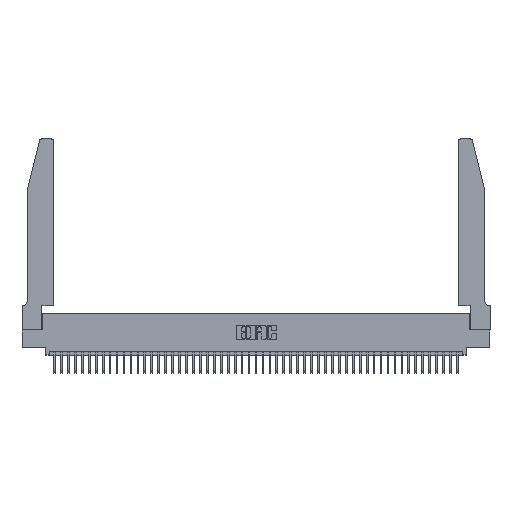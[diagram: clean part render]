
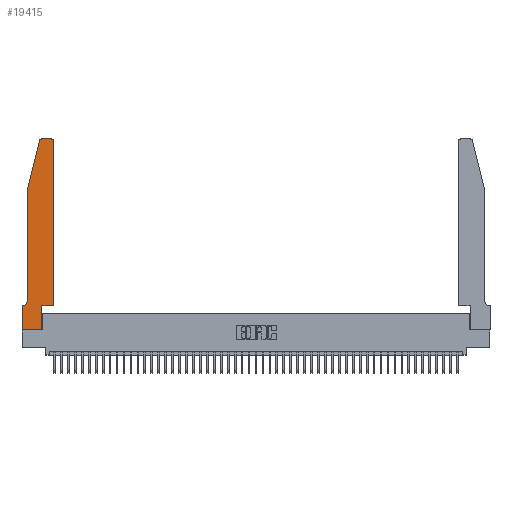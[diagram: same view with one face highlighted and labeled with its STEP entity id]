
A CAD part, top view. The second image highlights one B-rep face of the part: STEP entity #19415.
In plain terms, the highlighted planar face has unit normal (0, 0, 1).
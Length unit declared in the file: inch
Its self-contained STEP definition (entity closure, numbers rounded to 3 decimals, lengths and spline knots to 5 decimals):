
#170 = DIRECTION ( 'NONE',  ( 0., 0., -1. ) ) ;
#176 = LINE ( 'NONE', #2012, #18514 ) ;
#1061 = AXIS2_PLACEMENT_3D ( 'NONE', #16081, #1501, #27009 ) ;
#1501 = DIRECTION ( 'NONE',  ( 0., 0., 1. ) ) ;
#1616 = LINE ( 'NONE', #40275, #22205 ) ;
#2012 = CARTESIAN_POINT ( 'NONE',  ( 0.4505, 0.35, 0.37 ) ) ;
#2305 = CIRCLE ( 'NONE', #4295, 0.03 ) ;
#4044 = DIRECTION ( 'NONE',  ( 0., -1., 0. ) ) ;
#4295 = AXIS2_PLACEMENT_3D ( 'NONE', #20506, #45767, #24117 ) ;
#4886 = CARTESIAN_POINT ( 'NONE',  ( 0.2865, 0., 0.37 ) ) ;
#4923 = AXIS2_PLACEMENT_3D ( 'NONE', #7612, #32994, #11314 ) ;
#5019 = VECTOR ( 'NONE', #9269, 39.37008 ) ;
#5200 = EDGE_CURVE ( 'NONE', #31402, #45192, #18399, .T. ) ;
#5602 = VECTOR ( 'NONE', #7024, 39.37008 ) ;
#5701 = DIRECTION ( 'NONE',  ( 0., 1., 0. ) ) ;
#5814 = CARTESIAN_POINT ( 'NONE',  ( 0.284, 2.75, 0.37 ) ) ;
#6176 = CARTESIAN_POINT ( 'NONE',  ( 0.4505, 0.35, 0.37 ) ) ;
#6212 = LINE ( 'NONE', #27717, #43714 ) ;
#6852 = VECTOR ( 'NONE', #39383, 39.37008 ) ;
#6983 = DIRECTION ( 'NONE',  ( 0., -1., 0. ) ) ;
#7024 = DIRECTION ( 'NONE',  ( 1., 0., 0. ) ) ;
#7288 = VECTOR ( 'NONE', #44026, 39.37008 ) ;
#7612 = CARTESIAN_POINT ( 'NONE',  ( 0.4205, 2.72, 0.37 ) ) ;
#7862 = VERTEX_POINT ( 'NONE', #33078 ) ;
#8206 = VERTEX_POINT ( 'NONE', #4886 ) ;
#8473 = VERTEX_POINT ( 'NONE', #6176 ) ;
#8536 = ORIENTED_EDGE ( 'NONE', *, *, #20862, .T. ) ;
#8969 = VERTEX_POINT ( 'NONE', #5814 ) ;
#9269 = DIRECTION ( 'NONE',  ( -0.239, -0.971, 0. ) ) ;
#10121 = EDGE_CURVE ( 'NONE', #8473, #31402, #176, .T. ) ;
#10171 = VERTEX_POINT ( 'NONE', #24036 ) ;
#10353 = AXIS2_PLACEMENT_3D ( 'NONE', #22074, #170, #25716 ) ;
#11246 = ORIENTED_EDGE ( 'NONE', *, *, #12924, .T. ) ;
#11314 = DIRECTION ( 'NONE',  ( 1., 0., 0. ) ) ;
#11474 = CARTESIAN_POINT ( 'NONE',  ( 0., 0., 0.37 ) ) ;
#12151 = VERTEX_POINT ( 'NONE', #21371 ) ;
#12924 = EDGE_CURVE ( 'NONE', #27675, #14498, #1616, .T. ) ;
#13652 = EDGE_CURVE ( 'NONE', #12151, #8473, #18174, .T. ) ;
#13920 = EDGE_CURVE ( 'NONE', #10171, #21933, #14808, .T. ) ;
#14227 = CARTESIAN_POINT ( 'NONE',  ( 0.4505, 2.72, 0.37 ) ) ;
#14498 = VERTEX_POINT ( 'NONE', #11474 ) ;
#14808 = LINE ( 'NONE', #38283, #5019 ) ;
#15218 = ORIENTED_EDGE ( 'NONE', *, *, #5200, .T. ) ;
#15724 = CARTESIAN_POINT ( 'NONE',  ( 0., 0.35, 0.37 ) ) ;
#16081 = CARTESIAN_POINT ( 'NONE',  ( 0., 0.35, 0.37 ) ) ;
#16499 = LINE ( 'NONE', #39571, #5602 ) ;
#16736 = DIRECTION ( 'NONE',  ( 0., 1., 0. ) ) ;
#18174 = LINE ( 'NONE', #40362, #7288 ) ;
#18399 = CIRCLE ( 'NONE', #4923, 0.03 ) ;
#18514 = VECTOR ( 'NONE', #5701, 39.37008 ) ;
#19034 = EDGE_CURVE ( 'NONE', #21933, #22477, #36593, .T. ) ;
#19415 = ADVANCED_FACE ( 'NONE', ( #31479 ), #19753, .T. ) ;
#19580 = ORIENTED_EDGE ( 'NONE', *, *, #13920, .T. ) ;
#19753 = PLANE ( 'NONE',  #1061 ) ;
#20506 = CARTESIAN_POINT ( 'NONE',  ( 0.284, 2.72, 0.37 ) ) ;
#20862 = EDGE_CURVE ( 'NONE', #22477, #7862, #27941, .T. ) ;
#21371 = CARTESIAN_POINT ( 'NONE',  ( 0.2865, 0.35, 0.37 ) ) ;
#21933 = VERTEX_POINT ( 'NONE', #27657 ) ;
#22074 = CARTESIAN_POINT ( 'NONE',  ( 0.0055, 0.42, 0.37 ) ) ;
#22205 = VECTOR ( 'NONE', #4044, 39.37008 ) ;
#22477 = VERTEX_POINT ( 'NONE', #35037 ) ;
#23399 = ORIENTED_EDGE ( 'NONE', *, *, #19034, .T. ) ;
#23613 = LINE ( 'NONE', #27491, #32541 ) ;
#24036 = CARTESIAN_POINT ( 'NONE',  ( 0.25487, 2.72718, 0.37 ) ) ;
#24093 = DIRECTION ( 'NONE',  ( -1., 0., 0. ) ) ;
#24117 = DIRECTION ( 'NONE',  ( 1., 0., 0. ) ) ;
#24956 = EDGE_CURVE ( 'NONE', #8969, #10171, #2305, .T. ) ;
#25716 = DIRECTION ( 'NONE',  ( -1., 0., 0. ) ) ;
#26487 = CARTESIAN_POINT ( 'NONE',  ( 0.4205, 2.75, 0.37 ) ) ;
#27002 = VECTOR ( 'NONE', #6983, 39.37008 ) ;
#27009 = DIRECTION ( 'NONE',  ( 1., 0., 0. ) ) ;
#27491 = CARTESIAN_POINT ( 'NONE',  ( 0.2865, 0.35, 0.37 ) ) ;
#27657 = CARTESIAN_POINT ( 'NONE',  ( 0.0755, 2., 0.37 ) ) ;
#27675 = VERTEX_POINT ( 'NONE', #15724 ) ;
#27717 = CARTESIAN_POINT ( 'NONE',  ( 0.0755, 0.35, 0.37 ) ) ;
#27941 = CIRCLE ( 'NONE', #10353, 0.07 ) ;
#28866 = EDGE_CURVE ( 'NONE', #45192, #8969, #35806, .T. ) ;
#31133 = ORIENTED_EDGE ( 'NONE', *, *, #24956, .T. ) ;
#31401 = EDGE_LOOP ( 'NONE', ( #39023, #31133, #19580, #23399, #8536, #44535, #11246, #35185, #36945, #32228, #39153, #15218 ) ) ;
#31402 = VERTEX_POINT ( 'NONE', #14227 ) ;
#31479 = FACE_OUTER_BOUND ( 'NONE', #31401, .T. ) ;
#32228 = ORIENTED_EDGE ( 'NONE', *, *, #13652, .T. ) ;
#32541 = VECTOR ( 'NONE', #16736, 39.37008 ) ;
#32994 = DIRECTION ( 'NONE',  ( 0., 0., 1. ) ) ;
#33078 = CARTESIAN_POINT ( 'NONE',  ( 0.0055, 0.35, 0.37 ) ) ;
#35037 = CARTESIAN_POINT ( 'NONE',  ( 0.0755, 0.42, 0.37 ) ) ;
#35185 = ORIENTED_EDGE ( 'NONE', *, *, #40496, .T. ) ;
#35724 = CARTESIAN_POINT ( 'NONE',  ( 0.2605, 2.75, 0.37 ) ) ;
#35806 = LINE ( 'NONE', #35724, #6852 ) ;
#36593 = LINE ( 'NONE', #43193, #27002 ) ;
#36945 = ORIENTED_EDGE ( 'NONE', *, *, #37867, .T. ) ;
#37867 = EDGE_CURVE ( 'NONE', #8206, #12151, #23613, .T. ) ;
#38283 = CARTESIAN_POINT ( 'NONE',  ( 0.0755, 2., 0.37 ) ) ;
#39023 = ORIENTED_EDGE ( 'NONE', *, *, #28866, .T. ) ;
#39153 = ORIENTED_EDGE ( 'NONE', *, *, #10121, .T. ) ;
#39383 = DIRECTION ( 'NONE',  ( -1., 0., 0. ) ) ;
#39571 = CARTESIAN_POINT ( 'NONE',  ( 0., 0., 0.37 ) ) ;
#40275 = CARTESIAN_POINT ( 'NONE',  ( 0., 0., 0.37 ) ) ;
#40287 = EDGE_CURVE ( 'NONE', #7862, #27675, #6212, .T. ) ;
#40362 = CARTESIAN_POINT ( 'NONE',  ( 0.4505, 0.35, 0.37 ) ) ;
#40496 = EDGE_CURVE ( 'NONE', #14498, #8206, #16499, .T. ) ;
#43193 = CARTESIAN_POINT ( 'NONE',  ( 0.0755, 2., 0.37 ) ) ;
#43714 = VECTOR ( 'NONE', #24093, 39.37008 ) ;
#44026 = DIRECTION ( 'NONE',  ( 1., 0., 0. ) ) ;
#44535 = ORIENTED_EDGE ( 'NONE', *, *, #40287, .T. ) ;
#45192 = VERTEX_POINT ( 'NONE', #26487 ) ;
#45767 = DIRECTION ( 'NONE',  ( 0., 0., 1. ) ) ;
